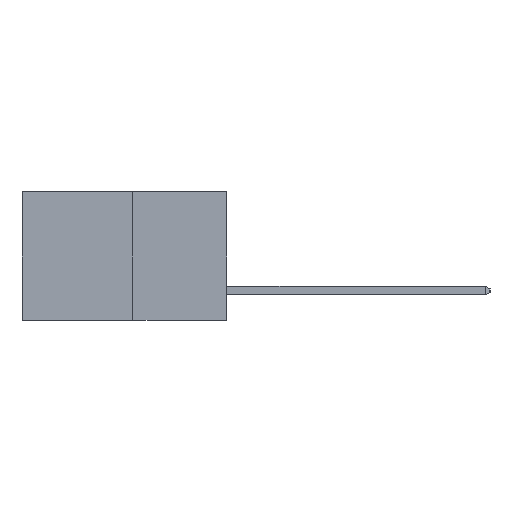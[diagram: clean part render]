
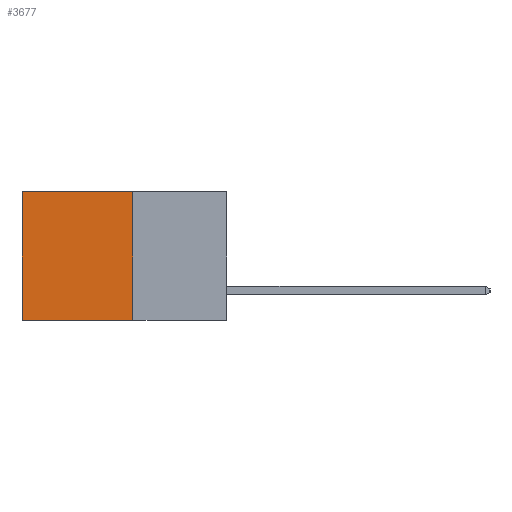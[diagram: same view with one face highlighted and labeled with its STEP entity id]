
A CAD part, left-side view. The second image highlights one B-rep face of the part: STEP entity #3677.
In plain terms, the highlighted planar face has unit normal (-1, 0, 0).
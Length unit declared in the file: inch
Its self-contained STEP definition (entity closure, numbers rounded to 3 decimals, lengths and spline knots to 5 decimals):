
#1505 = EDGE_CURVE ( 'NONE', #6163, #18303, #2932, .T. ) ;
#1852 = CARTESIAN_POINT ( 'NONE',  ( 0.277, 0.27, -0.37 ) ) ;
#2168 = VECTOR ( 'NONE', #22865, 39.37008 ) ;
#2173 = FACE_OUTER_BOUND ( 'NONE', #8271, .T. ) ;
#2932 = LINE ( 'NONE', #6623, #17832 ) ;
#3677 = ADVANCED_FACE ( 'NONE', ( #2173 ), #19926, .F. ) ;
#4137 = ORIENTED_EDGE ( 'NONE', *, *, #23584, .T. ) ;
#6163 = VERTEX_POINT ( 'NONE', #6258 ) ;
#6258 = CARTESIAN_POINT ( 'NONE',  ( 0.277, 0.59, 0. ) ) ;
#6623 = CARTESIAN_POINT ( 'NONE',  ( 0.277, 0.59, -0.37 ) ) ;
#8271 = EDGE_LOOP ( 'NONE', ( #17899, #13504, #13591, #4137 ) ) ;
#8517 = CARTESIAN_POINT ( 'NONE',  ( 0.277, 0.27, 0. ) ) ;
#8985 = CARTESIAN_POINT ( 'NONE',  ( 0.277, 0.27, 0. ) ) ;
#9321 = DIRECTION ( 'NONE',  ( 0., 0., -1. ) ) ;
#10250 = VECTOR ( 'NONE', #12107, 39.37008 ) ;
#10761 = CARTESIAN_POINT ( 'NONE',  ( 0.277, 0.27, -0.37 ) ) ;
#10787 = LINE ( 'NONE', #25699, #20127 ) ;
#12107 = DIRECTION ( 'NONE',  ( 0., 1., 0. ) ) ;
#13504 = ORIENTED_EDGE ( 'NONE', *, *, #21971, .F. ) ;
#13591 = ORIENTED_EDGE ( 'NONE', *, *, #16459, .F. ) ;
#14944 = CARTESIAN_POINT ( 'NONE',  ( 0.277, 0.27, -0.37 ) ) ;
#15042 = CARTESIAN_POINT ( 'NONE',  ( 0.277, 0.59, -0.37 ) ) ;
#15563 = LINE ( 'NONE', #1852, #10250 ) ;
#16207 = DIRECTION ( 'NONE',  ( 1., 0., 0. ) ) ;
#16232 = DIRECTION ( 'NONE',  ( 0., 0., -1. ) ) ;
#16459 = EDGE_CURVE ( 'NONE', #25191, #24061, #10787, .T. ) ;
#17181 = AXIS2_PLACEMENT_3D ( 'NONE', #14944, #16207, #16232 ) ;
#17703 = LINE ( 'NONE', #8985, #2168 ) ;
#17832 = VECTOR ( 'NONE', #9321, 39.37008 ) ;
#17899 = ORIENTED_EDGE ( 'NONE', *, *, #1505, .T. ) ;
#17907 = DIRECTION ( 'NONE',  ( 0., 0., -1. ) ) ;
#18303 = VERTEX_POINT ( 'NONE', #15042 ) ;
#19926 = PLANE ( 'NONE',  #17181 ) ;
#20127 = VECTOR ( 'NONE', #17907, 39.37008 ) ;
#21971 = EDGE_CURVE ( 'NONE', #24061, #18303, #15563, .T. ) ;
#22865 = DIRECTION ( 'NONE',  ( 0., 1., 0. ) ) ;
#23584 = EDGE_CURVE ( 'NONE', #25191, #6163, #17703, .T. ) ;
#24061 = VERTEX_POINT ( 'NONE', #10761 ) ;
#25191 = VERTEX_POINT ( 'NONE', #8517 ) ;
#25699 = CARTESIAN_POINT ( 'NONE',  ( 0.277, 0.27, -0.37 ) ) ;
